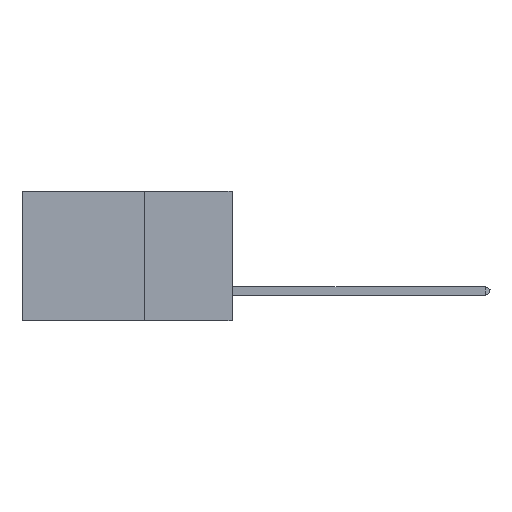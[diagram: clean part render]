
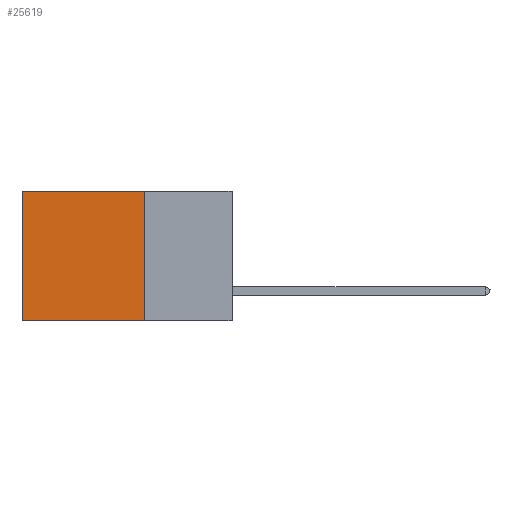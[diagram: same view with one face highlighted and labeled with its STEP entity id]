
A CAD part, left-side view. The second image highlights one B-rep face of the part: STEP entity #25619.
In plain terms, the highlighted planar face has unit normal (-1, 0, 0).
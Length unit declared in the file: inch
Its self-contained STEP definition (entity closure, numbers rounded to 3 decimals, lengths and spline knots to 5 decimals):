
#454 = CARTESIAN_POINT ( 'NONE',  ( 0.2875, 0.6, -0.37 ) ) ;
#828 = ORIENTED_EDGE ( 'NONE', *, *, #28414, .T. ) ;
#1734 = EDGE_CURVE ( 'NONE', #18940, #26705, #17440, .T. ) ;
#2723 = ORIENTED_EDGE ( 'NONE', *, *, #28727, .T. ) ;
#2996 = CARTESIAN_POINT ( 'NONE',  ( 0.2875, 0.25, 0. ) ) ;
#4431 = DIRECTION ( 'NONE',  ( 0., 1., 0. ) ) ;
#5324 = LINE ( 'NONE', #23299, #24913 ) ;
#8093 = VECTOR ( 'NONE', #23325, 39.37008 ) ;
#9728 = EDGE_CURVE ( 'NONE', #14183, #18940, #5324, .T. ) ;
#9834 = DIRECTION ( 'NONE',  ( 0., 0., -1. ) ) ;
#10774 = EDGE_LOOP ( 'NONE', ( #2723, #13326, #27724, #828 ) ) ;
#10798 = VECTOR ( 'NONE', #21490, 39.37008 ) ;
#13242 = CARTESIAN_POINT ( 'NONE',  ( 0.2875, 0.25, 0. ) ) ;
#13326 = ORIENTED_EDGE ( 'NONE', *, *, #1734, .F. ) ;
#13484 = CARTESIAN_POINT ( 'NONE',  ( 0.2875, 0.25, 0. ) ) ;
#14183 = VERTEX_POINT ( 'NONE', #13484 ) ;
#14206 = DIRECTION ( 'NONE',  ( 1., 0., 0. ) ) ;
#15427 = CARTESIAN_POINT ( 'NONE',  ( 0.2875, 0.6, 0. ) ) ;
#15938 = CARTESIAN_POINT ( 'NONE',  ( 0.2875, 0.25, -0.37 ) ) ;
#17440 = LINE ( 'NONE', #15938, #10798 ) ;
#17562 = LINE ( 'NONE', #27361, #8093 ) ;
#18695 = DIRECTION ( 'NONE',  ( 0., 0., -1. ) ) ;
#18789 = PLANE ( 'NONE',  #27845 ) ;
#18940 = VERTEX_POINT ( 'NONE', #25366 ) ;
#19315 = VECTOR ( 'NONE', #4431, 39.37008 ) ;
#21039 = VERTEX_POINT ( 'NONE', #15427 ) ;
#21490 = DIRECTION ( 'NONE',  ( 0., 1., 0. ) ) ;
#21753 = LINE ( 'NONE', #13242, #19315 ) ;
#23299 = CARTESIAN_POINT ( 'NONE',  ( 0.2875, 0.25, 0. ) ) ;
#23325 = DIRECTION ( 'NONE',  ( 0., 0., -1. ) ) ;
#24913 = VECTOR ( 'NONE', #9834, 39.37008 ) ;
#25366 = CARTESIAN_POINT ( 'NONE',  ( 0.2875, 0.25, -0.37 ) ) ;
#25619 = ADVANCED_FACE ( 'NONE', ( #27653 ), #18789, .F. ) ;
#26705 = VERTEX_POINT ( 'NONE', #454 ) ;
#27361 = CARTESIAN_POINT ( 'NONE',  ( 0.2875, 0.6, 0. ) ) ;
#27653 = FACE_OUTER_BOUND ( 'NONE', #10774, .T. ) ;
#27724 = ORIENTED_EDGE ( 'NONE', *, *, #9728, .F. ) ;
#27845 = AXIS2_PLACEMENT_3D ( 'NONE', #2996, #14206, #18695 ) ;
#28414 = EDGE_CURVE ( 'NONE', #14183, #21039, #21753, .T. ) ;
#28727 = EDGE_CURVE ( 'NONE', #21039, #26705, #17562, .T. ) ;
